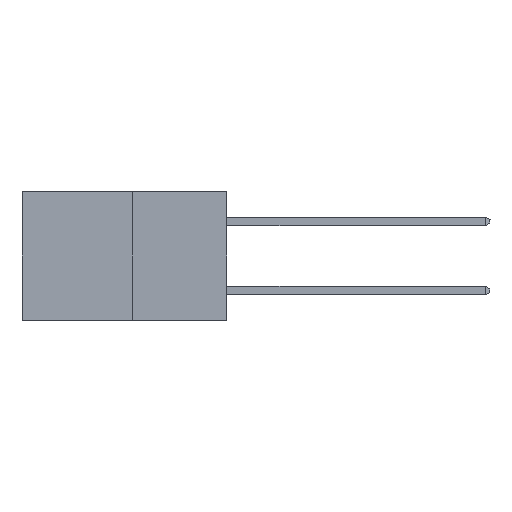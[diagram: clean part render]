
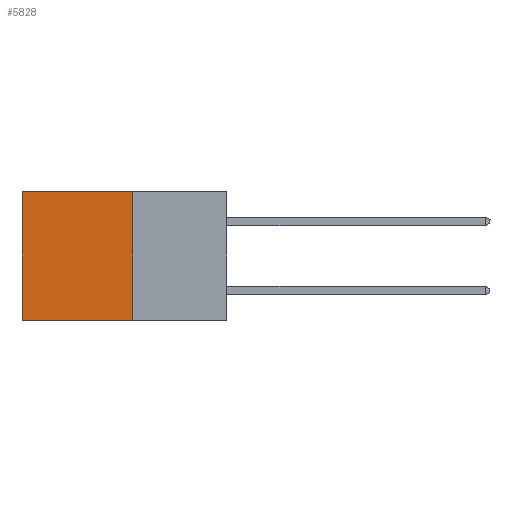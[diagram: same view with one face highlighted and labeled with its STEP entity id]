
A CAD part, left-side view. The second image highlights one B-rep face of the part: STEP entity #5828.
In plain terms, the highlighted planar face has unit normal (-1, 0, 0).
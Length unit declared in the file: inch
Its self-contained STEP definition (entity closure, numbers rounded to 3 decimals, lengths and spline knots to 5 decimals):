
#274 = CARTESIAN_POINT ( 'NONE',  ( 0.277, 0.27, 0. ) ) ;
#381 = CARTESIAN_POINT ( 'NONE',  ( 0.277, 0.27, 0. ) ) ;
#828 = AXIS2_PLACEMENT_3D ( 'NONE', #13997, #11480, #4961 ) ;
#1131 = DIRECTION ( 'NONE',  ( 0., 1., 0. ) ) ;
#2047 = LINE ( 'NONE', #11632, #10896 ) ;
#2513 = CARTESIAN_POINT ( 'NONE',  ( 0.277, 0.27, -0.37 ) ) ;
#2728 = VECTOR ( 'NONE', #12822, 39.37008 ) ;
#2783 = EDGE_CURVE ( 'NONE', #4584, #11373, #2047, .T. ) ;
#4391 = LINE ( 'NONE', #14005, #13094 ) ;
#4584 = VERTEX_POINT ( 'NONE', #5702 ) ;
#4769 = VERTEX_POINT ( 'NONE', #7000 ) ;
#4961 = DIRECTION ( 'NONE',  ( 0., 0., -1. ) ) ;
#5160 = EDGE_CURVE ( 'NONE', #8239, #4769, #14499, .T. ) ;
#5702 = CARTESIAN_POINT ( 'NONE',  ( 0.277, 0.59, 0. ) ) ;
#5828 = ADVANCED_FACE ( 'NONE', ( #10611 ), #14464, .F. ) ;
#6816 = EDGE_CURVE ( 'NONE', #8239, #4584, #10583, .T. ) ;
#7000 = CARTESIAN_POINT ( 'NONE',  ( 0.277, 0.27, -0.37 ) ) ;
#7084 = ORIENTED_EDGE ( 'NONE', *, *, #6816, .T. ) ;
#7602 = VECTOR ( 'NONE', #1131, 39.37008 ) ;
#7699 = CARTESIAN_POINT ( 'NONE',  ( 0.277, 0.59, -0.37 ) ) ;
#7930 = ORIENTED_EDGE ( 'NONE', *, *, #11865, .F. ) ;
#8239 = VERTEX_POINT ( 'NONE', #381 ) ;
#8317 = DIRECTION ( 'NONE',  ( 0., 0., -1. ) ) ;
#10583 = LINE ( 'NONE', #274, #7602 ) ;
#10611 = FACE_OUTER_BOUND ( 'NONE', #14437, .T. ) ;
#10896 = VECTOR ( 'NONE', #8317, 39.37008 ) ;
#11373 = VERTEX_POINT ( 'NONE', #7699 ) ;
#11480 = DIRECTION ( 'NONE',  ( 1., 0., 0. ) ) ;
#11632 = CARTESIAN_POINT ( 'NONE',  ( 0.277, 0.59, -0.37 ) ) ;
#11865 = EDGE_CURVE ( 'NONE', #4769, #11373, #4391, .T. ) ;
#12822 = DIRECTION ( 'NONE',  ( 0., 0., -1. ) ) ;
#12862 = DIRECTION ( 'NONE',  ( 0., 1., 0. ) ) ;
#13094 = VECTOR ( 'NONE', #12862, 39.37008 ) ;
#13572 = ORIENTED_EDGE ( 'NONE', *, *, #2783, .T. ) ;
#13949 = ORIENTED_EDGE ( 'NONE', *, *, #5160, .F. ) ;
#13997 = CARTESIAN_POINT ( 'NONE',  ( 0.277, 0.27, -0.37 ) ) ;
#14005 = CARTESIAN_POINT ( 'NONE',  ( 0.277, 0.27, -0.37 ) ) ;
#14437 = EDGE_LOOP ( 'NONE', ( #13572, #7930, #13949, #7084 ) ) ;
#14464 = PLANE ( 'NONE',  #828 ) ;
#14499 = LINE ( 'NONE', #2513, #2728 ) ;
